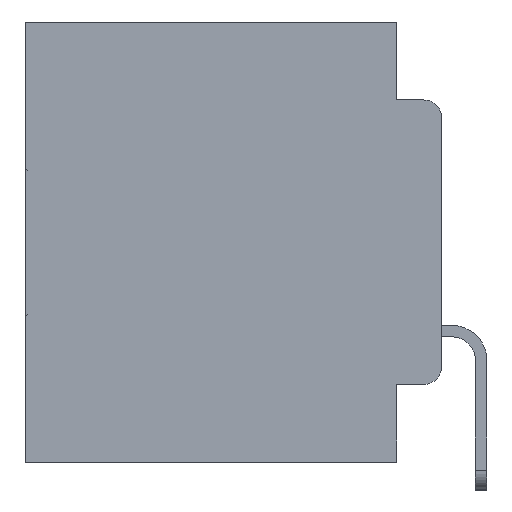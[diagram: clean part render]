
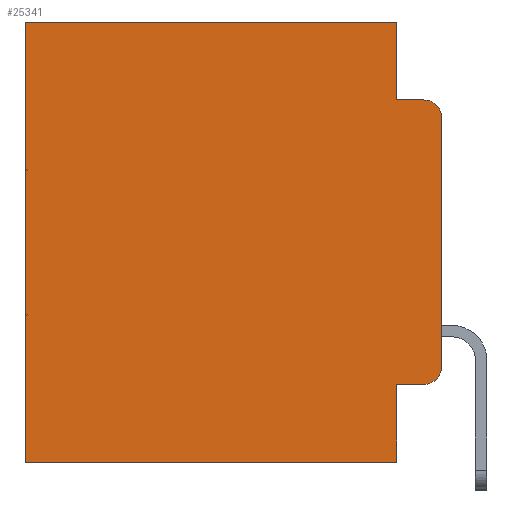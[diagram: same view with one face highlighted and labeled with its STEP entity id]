
A CAD part, left-side view. The second image highlights one B-rep face of the part: STEP entity #25341.
In plain terms, the highlighted planar face has unit normal (-1, 0, 0).
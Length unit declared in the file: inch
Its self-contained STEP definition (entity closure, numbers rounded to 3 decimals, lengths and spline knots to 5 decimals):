
#622 = ORIENTED_EDGE ( 'NONE', *, *, #16130, .T. ) ;
#2529 = AXIS2_PLACEMENT_3D ( 'NONE', #28932, #30205, #22797 ) ;
#2576 = ORIENTED_EDGE ( 'NONE', *, *, #5285, .F. ) ;
#2840 = DIRECTION ( 'NONE',  ( 0., 1., 0. ) ) ;
#3902 = CARTESIAN_POINT ( 'NONE',  ( 0.298, 0.02, -0.4115 ) ) ;
#4005 = DIRECTION ( 'NONE',  ( 0., 1., 0. ) ) ;
#4171 = CIRCLE ( 'NONE', #15324, 0.02 ) ;
#4316 = FACE_OUTER_BOUND ( 'NONE', #23885, .T. ) ;
#4571 = DIRECTION ( 'NONE',  ( 0., 0., -1. ) ) ;
#5285 = EDGE_CURVE ( 'NONE', #25537, #10933, #13808, .T. ) ;
#5300 = EDGE_CURVE ( 'NONE', #30597, #10695, #24579, .T. ) ;
#5467 = CARTESIAN_POINT ( 'NONE',  ( 0.298, 0.051, -0.5 ) ) ;
#5725 = ORIENTED_EDGE ( 'NONE', *, *, #13638, .T. ) ;
#5827 = AXIS2_PLACEMENT_3D ( 'NONE', #27072, #12987, #8308 ) ;
#6421 = ORIENTED_EDGE ( 'NONE', *, *, #8787, .T. ) ;
#6530 = DIRECTION ( 'NONE',  ( -1., 0., 0. ) ) ;
#7124 = DIRECTION ( 'NONE',  ( 0., 0., -1. ) ) ;
#7217 = DIRECTION ( 'NONE',  ( 0., 0., -1. ) ) ;
#7240 = LINE ( 'NONE', #21752, #24969 ) ;
#8308 = DIRECTION ( 'NONE',  ( 0., 0., -1. ) ) ;
#8500 = VECTOR ( 'NONE', #27274, 39.37008 ) ;
#8787 = EDGE_CURVE ( 'NONE', #23511, #16745, #19131, .T. ) ;
#8967 = CARTESIAN_POINT ( 'NONE',  ( 0.298, 0.473, -0.5 ) ) ;
#9411 = VECTOR ( 'NONE', #4005, 39.37008 ) ;
#10695 = VERTEX_POINT ( 'NONE', #5467 ) ;
#10757 = VECTOR ( 'NONE', #29118, 39.37008 ) ;
#10933 = VERTEX_POINT ( 'NONE', #11005 ) ;
#11005 = CARTESIAN_POINT ( 'NONE',  ( 0.298, 0.051, -0.0885 ) ) ;
#11011 = CARTESIAN_POINT ( 'NONE',  ( 0.298, 0.051, -0.4115 ) ) ;
#11103 = LINE ( 'NONE', #21254, #23701 ) ;
#11993 = CARTESIAN_POINT ( 'NONE',  ( 0.298, 0.051, 0. ) ) ;
#12254 = CARTESIAN_POINT ( 'NONE',  ( 0.298, 0., 0. ) ) ;
#12363 = VERTEX_POINT ( 'NONE', #13202 ) ;
#12987 = DIRECTION ( 'NONE',  ( 1., 0., 0. ) ) ;
#13202 = CARTESIAN_POINT ( 'NONE',  ( 0.298, 0.473, 0. ) ) ;
#13546 = EDGE_CURVE ( 'NONE', #23511, #23237, #28153, .T. ) ;
#13638 = EDGE_CURVE ( 'NONE', #30597, #26448, #15150, .T. ) ;
#13732 = CARTESIAN_POINT ( 'NONE',  ( 0.298, 0.051, -0.4115 ) ) ;
#13808 = LINE ( 'NONE', #18921, #16011 ) ;
#13880 = EDGE_CURVE ( 'NONE', #12363, #20673, #11103, .T. ) ;
#15150 = LINE ( 'NONE', #11011, #8500 ) ;
#15222 = DIRECTION ( 'NONE',  ( 0., -1., 0. ) ) ;
#15324 = AXIS2_PLACEMENT_3D ( 'NONE', #30135, #6530, #23129 ) ;
#15597 = CARTESIAN_POINT ( 'NONE',  ( 0.298, 0., -0.1085 ) ) ;
#15726 = EDGE_CURVE ( 'NONE', #10933, #16745, #7240, .T. ) ;
#15876 = CARTESIAN_POINT ( 'NONE',  ( 0.298, 0., -0.5 ) ) ;
#16011 = VECTOR ( 'NONE', #7124, 39.37008 ) ;
#16130 = EDGE_CURVE ( 'NONE', #26448, #23237, #4171, .T. ) ;
#16745 = VERTEX_POINT ( 'NONE', #24027 ) ;
#17745 = ORIENTED_EDGE ( 'NONE', *, *, #26511, .F. ) ;
#17856 = ORIENTED_EDGE ( 'NONE', *, *, #13546, .F. ) ;
#18043 = VECTOR ( 'NONE', #2840, 39.37008 ) ;
#18921 = CARTESIAN_POINT ( 'NONE',  ( 0.298, 0.051, 0. ) ) ;
#19131 = CIRCLE ( 'NONE', #2529, 0.02 ) ;
#20673 = VERTEX_POINT ( 'NONE', #8967 ) ;
#21254 = CARTESIAN_POINT ( 'NONE',  ( 0.298, 0.473, 0. ) ) ;
#21752 = CARTESIAN_POINT ( 'NONE',  ( 0.298, 0.051, -0.0885 ) ) ;
#21864 = CARTESIAN_POINT ( 'NONE',  ( 0.298, 0., -0.3915 ) ) ;
#21891 = ORIENTED_EDGE ( 'NONE', *, *, #13880, .T. ) ;
#22797 = DIRECTION ( 'NONE',  ( 0., 0., -1. ) ) ;
#23129 = DIRECTION ( 'NONE',  ( 0., 0., -1. ) ) ;
#23237 = VERTEX_POINT ( 'NONE', #21864 ) ;
#23511 = VERTEX_POINT ( 'NONE', #15597 ) ;
#23701 = VECTOR ( 'NONE', #4571, 39.37008 ) ;
#23885 = EDGE_LOOP ( 'NONE', ( #17856, #6421, #24981, #2576, #29992, #21891, #17745, #28159, #5725, #622 ) ) ;
#24027 = CARTESIAN_POINT ( 'NONE',  ( 0.298, 0.02, -0.0885 ) ) ;
#24362 = LINE ( 'NONE', #12254, #18043 ) ;
#24376 = CARTESIAN_POINT ( 'NONE',  ( 0.298, 0., 0. ) ) ;
#24579 = LINE ( 'NONE', #11993, #30465 ) ;
#24969 = VECTOR ( 'NONE', #15222, 39.37008 ) ;
#24981 = ORIENTED_EDGE ( 'NONE', *, *, #15726, .F. ) ;
#25077 = EDGE_CURVE ( 'NONE', #25537, #12363, #24362, .T. ) ;
#25341 = ADVANCED_FACE ( 'NONE', ( #4316 ), #27471, .F. ) ;
#25537 = VERTEX_POINT ( 'NONE', #25904 ) ;
#25904 = CARTESIAN_POINT ( 'NONE',  ( 0.298, 0.051, 0. ) ) ;
#26448 = VERTEX_POINT ( 'NONE', #3902 ) ;
#26511 = EDGE_CURVE ( 'NONE', #10695, #20673, #29032, .T. ) ;
#27072 = CARTESIAN_POINT ( 'NONE',  ( 0.298, 0., 0. ) ) ;
#27274 = DIRECTION ( 'NONE',  ( 0., -1., 0. ) ) ;
#27471 = PLANE ( 'NONE',  #5827 ) ;
#28153 = LINE ( 'NONE', #24376, #10757 ) ;
#28159 = ORIENTED_EDGE ( 'NONE', *, *, #5300, .F. ) ;
#28932 = CARTESIAN_POINT ( 'NONE',  ( 0.298, 0.02, -0.1085 ) ) ;
#29032 = LINE ( 'NONE', #15876, #9411 ) ;
#29118 = DIRECTION ( 'NONE',  ( 0., 0., -1. ) ) ;
#29992 = ORIENTED_EDGE ( 'NONE', *, *, #25077, .T. ) ;
#30135 = CARTESIAN_POINT ( 'NONE',  ( 0.298, 0.02, -0.3915 ) ) ;
#30205 = DIRECTION ( 'NONE',  ( -1., 0., 0. ) ) ;
#30465 = VECTOR ( 'NONE', #7217, 39.37008 ) ;
#30597 = VERTEX_POINT ( 'NONE', #13732 ) ;
